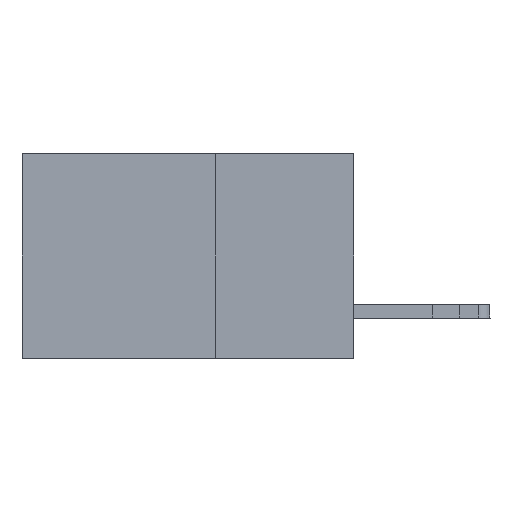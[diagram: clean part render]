
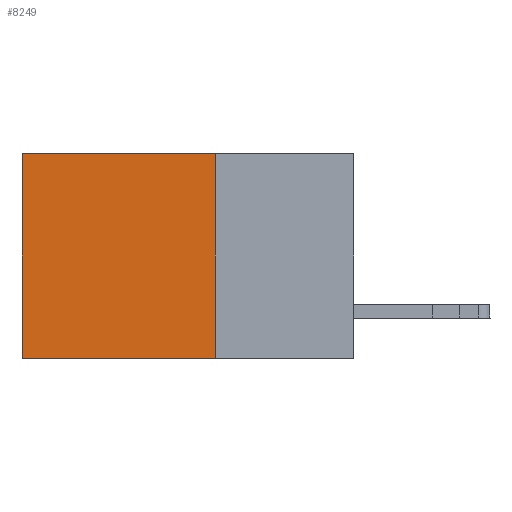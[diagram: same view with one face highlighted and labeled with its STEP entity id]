
A CAD part, left-side view. The second image highlights one B-rep face of the part: STEP entity #8249.
In plain terms, the highlighted planar face has unit normal (-1, 0, 0).
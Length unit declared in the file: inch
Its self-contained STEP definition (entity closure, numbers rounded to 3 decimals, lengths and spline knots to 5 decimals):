
#1905 = LINE ( 'NONE', #16037, #16667 ) ;
#4071 = DIRECTION ( 'NONE',  ( 0., 0., -1. ) ) ;
#4276 = DIRECTION ( 'NONE',  ( 0., 1., 0. ) ) ;
#5050 = PLANE ( 'NONE',  #24550 ) ;
#6283 = CARTESIAN_POINT ( 'NONE',  ( 0.2875, 0.6, -0.37 ) ) ;
#6812 = LINE ( 'NONE', #24704, #37369 ) ;
#8169 = ORIENTED_EDGE ( 'NONE', *, *, #37330, .F. ) ;
#8249 = ADVANCED_FACE ( 'NONE', ( #22415 ), #5050, .F. ) ;
#9304 = EDGE_CURVE ( 'NONE', #35078, #36511, #23875, .T. ) ;
#10969 = DIRECTION ( 'NONE',  ( 0., 0., -1. ) ) ;
#11904 = CARTESIAN_POINT ( 'NONE',  ( 0.2875, 0.6, 0. ) ) ;
#12004 = VECTOR ( 'NONE', #37495, 39.37008 ) ;
#14397 = VERTEX_POINT ( 'NONE', #6283 ) ;
#15996 = VECTOR ( 'NONE', #4071, 39.37008 ) ;
#16037 = CARTESIAN_POINT ( 'NONE',  ( 0.2875, 0.25, -0.37 ) ) ;
#16589 = EDGE_LOOP ( 'NONE', ( #19558, #8169, #18691, #24086 ) ) ;
#16667 = VECTOR ( 'NONE', #4276, 39.37008 ) ;
#16797 = CARTESIAN_POINT ( 'NONE',  ( 0.2875, 0.6, 0. ) ) ;
#18691 = ORIENTED_EDGE ( 'NONE', *, *, #9304, .F. ) ;
#19558 = ORIENTED_EDGE ( 'NONE', *, *, #37479, .T. ) ;
#20133 = EDGE_CURVE ( 'NONE', #35078, #35904, #6812, .T. ) ;
#21725 = DIRECTION ( 'NONE',  ( 0., 1., 0. ) ) ;
#22415 = FACE_OUTER_BOUND ( 'NONE', #16589, .T. ) ;
#23875 = LINE ( 'NONE', #36537, #15996 ) ;
#24086 = ORIENTED_EDGE ( 'NONE', *, *, #20133, .T. ) ;
#24550 = AXIS2_PLACEMENT_3D ( 'NONE', #25762, #28730, #10969 ) ;
#24704 = CARTESIAN_POINT ( 'NONE',  ( 0.2875, 0.25, 0. ) ) ;
#25762 = CARTESIAN_POINT ( 'NONE',  ( 0.2875, 0.25, 0. ) ) ;
#26381 = CARTESIAN_POINT ( 'NONE',  ( 0.2875, 0.25, -0.37 ) ) ;
#28730 = DIRECTION ( 'NONE',  ( 1., 0., 0. ) ) ;
#34618 = CARTESIAN_POINT ( 'NONE',  ( 0.2875, 0.25, 0. ) ) ;
#34705 = LINE ( 'NONE', #16797, #12004 ) ;
#35078 = VERTEX_POINT ( 'NONE', #34618 ) ;
#35904 = VERTEX_POINT ( 'NONE', #11904 ) ;
#36511 = VERTEX_POINT ( 'NONE', #26381 ) ;
#36537 = CARTESIAN_POINT ( 'NONE',  ( 0.2875, 0.25, 0. ) ) ;
#37330 = EDGE_CURVE ( 'NONE', #36511, #14397, #1905, .T. ) ;
#37369 = VECTOR ( 'NONE', #21725, 39.37008 ) ;
#37479 = EDGE_CURVE ( 'NONE', #35904, #14397, #34705, .T. ) ;
#37495 = DIRECTION ( 'NONE',  ( 0., 0., -1. ) ) ;
